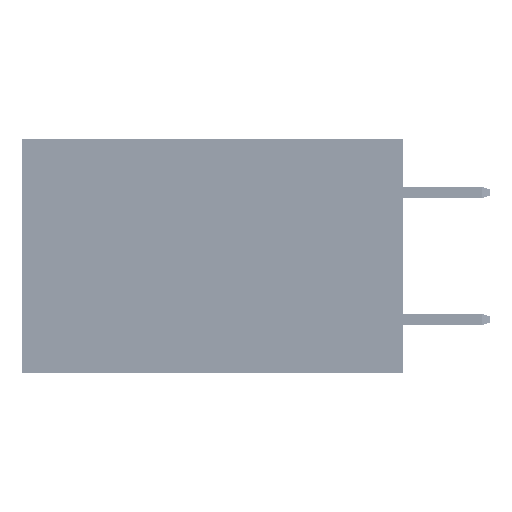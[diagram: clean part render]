
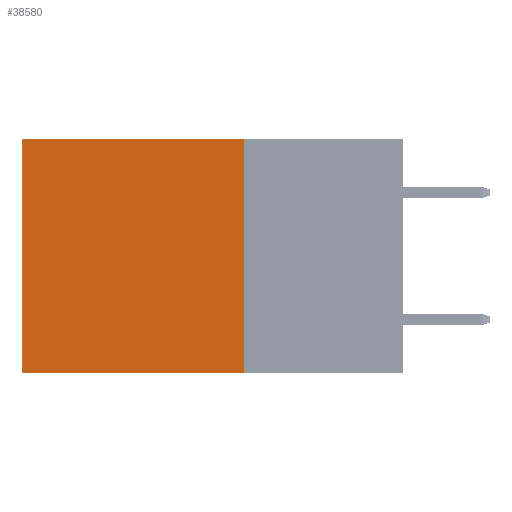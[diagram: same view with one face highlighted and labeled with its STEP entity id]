
A CAD part, left-side view. The second image highlights one B-rep face of the part: STEP entity #38580.
In plain terms, the highlighted planar face has unit normal (-1, 0, 0).
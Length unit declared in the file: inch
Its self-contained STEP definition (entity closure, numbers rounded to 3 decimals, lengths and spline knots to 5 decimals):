
#2590 = CARTESIAN_POINT ( 'NONE',  ( 0.2875, 0.6, 0. ) ) ;
#2619 = VERTEX_POINT ( 'NONE', #14070 ) ;
#4718 = LINE ( 'NONE', #9379, #38152 ) ;
#5145 = CARTESIAN_POINT ( 'NONE',  ( 0.2875, 0.25, -0.37 ) ) ;
#5214 = LINE ( 'NONE', #28810, #43033 ) ;
#9379 = CARTESIAN_POINT ( 'NONE',  ( 0.2875, 0.6, 0. ) ) ;
#13771 = EDGE_CURVE ( 'NONE', #26704, #27031, #4718, .T. ) ;
#14070 = CARTESIAN_POINT ( 'NONE',  ( 0.2875, 0.25, 0. ) ) ;
#14410 = AXIS2_PLACEMENT_3D ( 'NONE', #47496, #30452, #23364 ) ;
#15583 = CARTESIAN_POINT ( 'NONE',  ( 0.2875, 0.25, 0. ) ) ;
#17746 = ORIENTED_EDGE ( 'NONE', *, *, #42539, .F. ) ;
#18911 = ORIENTED_EDGE ( 'NONE', *, *, #23042, .F. ) ;
#23042 = EDGE_CURVE ( 'NONE', #48774, #27031, #29006, .T. ) ;
#23364 = DIRECTION ( 'NONE',  ( 0., 0., -1. ) ) ;
#26704 = VERTEX_POINT ( 'NONE', #2590 ) ;
#27031 = VERTEX_POINT ( 'NONE', #29004 ) ;
#28810 = CARTESIAN_POINT ( 'NONE',  ( 0.2875, 0.25, 0. ) ) ;
#29004 = CARTESIAN_POINT ( 'NONE',  ( 0.2875, 0.6, -0.37 ) ) ;
#29006 = LINE ( 'NONE', #5145, #44512 ) ;
#29769 = DIRECTION ( 'NONE',  ( 0., 1., 0. ) ) ;
#30452 = DIRECTION ( 'NONE',  ( 1., 0., 0. ) ) ;
#30462 = CARTESIAN_POINT ( 'NONE',  ( 0.2875, 0.25, -0.37 ) ) ;
#30576 = VECTOR ( 'NONE', #31338, 39.37008 ) ;
#31338 = DIRECTION ( 'NONE',  ( 0., 1., 0. ) ) ;
#33022 = DIRECTION ( 'NONE',  ( 0., 0., -1. ) ) ;
#34257 = DIRECTION ( 'NONE',  ( 0., 0., -1. ) ) ;
#37646 = EDGE_LOOP ( 'NONE', ( #40083, #18911, #17746, #50052 ) ) ;
#38152 = VECTOR ( 'NONE', #34257, 39.37008 ) ;
#38580 = ADVANCED_FACE ( 'NONE', ( #43311 ), #46727, .F. ) ;
#40083 = ORIENTED_EDGE ( 'NONE', *, *, #13771, .T. ) ;
#42539 = EDGE_CURVE ( 'NONE', #2619, #48774, #5214, .T. ) ;
#43033 = VECTOR ( 'NONE', #33022, 39.37008 ) ;
#43311 = FACE_OUTER_BOUND ( 'NONE', #37646, .T. ) ;
#44471 = EDGE_CURVE ( 'NONE', #2619, #26704, #48566, .T. ) ;
#44512 = VECTOR ( 'NONE', #29769, 39.37008 ) ;
#46727 = PLANE ( 'NONE',  #14410 ) ;
#47496 = CARTESIAN_POINT ( 'NONE',  ( 0.2875, 0.25, 0. ) ) ;
#48566 = LINE ( 'NONE', #15583, #30576 ) ;
#48774 = VERTEX_POINT ( 'NONE', #30462 ) ;
#50052 = ORIENTED_EDGE ( 'NONE', *, *, #44471, .T. ) ;
